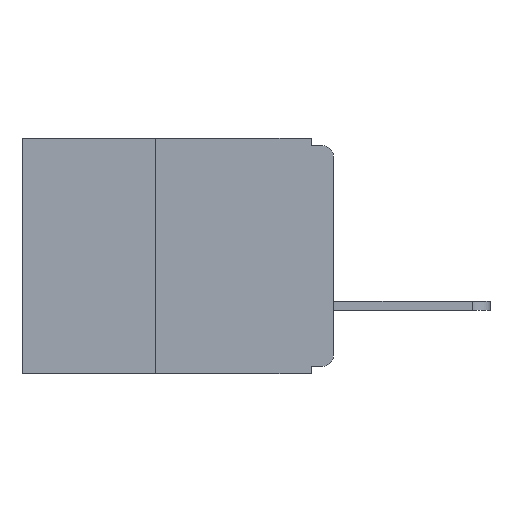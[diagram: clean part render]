
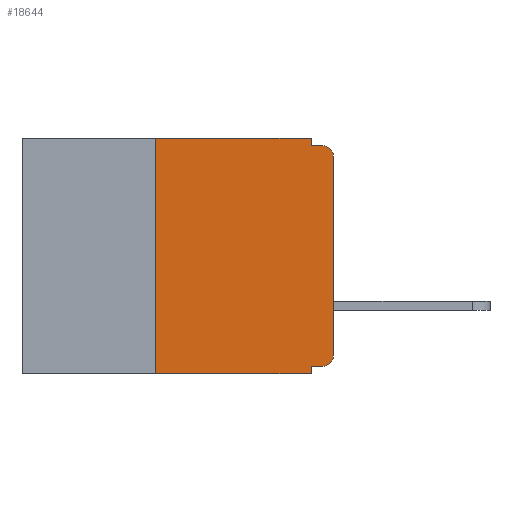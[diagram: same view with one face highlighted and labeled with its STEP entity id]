
A CAD part, left-side view. The second image highlights one B-rep face of the part: STEP entity #18644.
In plain terms, the highlighted planar face has unit normal (-1, 0, 0).
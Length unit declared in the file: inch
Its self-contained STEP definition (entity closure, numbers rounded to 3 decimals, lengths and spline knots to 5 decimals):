
#271 = VECTOR ( 'NONE', #26319, 39.37008 ) ;
#470 = EDGE_CURVE ( 'NONE', #30614, #11118, #21927, .T. ) ;
#960 = VECTOR ( 'NONE', #23253, 39.37008 ) ;
#1265 = VERTEX_POINT ( 'NONE', #15698 ) ;
#1333 = CARTESIAN_POINT ( 'NONE',  ( 0., 0.031, 0. ) ) ;
#3587 = DIRECTION ( 'NONE',  ( 0., 0., -1. ) ) ;
#4010 = DIRECTION ( 'NONE',  ( 0., 0., -1. ) ) ;
#4295 = EDGE_CURVE ( 'NONE', #5177, #17000, #7748, .T. ) ;
#4303 = CARTESIAN_POINT ( 'NONE',  ( 0., 0.015, -0.01 ) ) ;
#5177 = VERTEX_POINT ( 'NONE', #26913 ) ;
#5178 = LINE ( 'NONE', #8934, #17612 ) ;
#5213 = VECTOR ( 'NONE', #18638, 39.37008 ) ;
#6089 = CARTESIAN_POINT ( 'NONE',  ( 0., 0.031, -0.33 ) ) ;
#6335 = DIRECTION ( 'NONE',  ( 0., -1., 0. ) ) ;
#6690 = EDGE_CURVE ( 'NONE', #17000, #25596, #9589, .T. ) ;
#6810 = LINE ( 'NONE', #26213, #271 ) ;
#7748 = LINE ( 'NONE', #12153, #20123 ) ;
#7890 = EDGE_CURVE ( 'NONE', #17106, #25596, #20689, .T. ) ;
#8322 = FACE_OUTER_BOUND ( 'NONE', #29855, .T. ) ;
#8396 = CARTESIAN_POINT ( 'NONE',  ( 0., 0.25, -0.33 ) ) ;
#8934 = CARTESIAN_POINT ( 'NONE',  ( 0., 0.031, -0.33 ) ) ;
#9293 = ORIENTED_EDGE ( 'NONE', *, *, #21731, .T. ) ;
#9324 = CARTESIAN_POINT ( 'NONE',  ( 0., 0.015, -0.305 ) ) ;
#9589 = CIRCLE ( 'NONE', #30154, 0.015 ) ;
#10976 = CARTESIAN_POINT ( 'NONE',  ( 0., 0.437, 0. ) ) ;
#11118 = VERTEX_POINT ( 'NONE', #6089 ) ;
#11634 = LINE ( 'NONE', #28216, #24750 ) ;
#11778 = DIRECTION ( 'NONE',  ( 0., 0., -1. ) ) ;
#12010 = CARTESIAN_POINT ( 'NONE',  ( 0., 0.031, -0.32 ) ) ;
#12043 = DIRECTION ( 'NONE',  ( 0., 0., 1. ) ) ;
#12153 = CARTESIAN_POINT ( 'NONE',  ( 0., 0., 0. ) ) ;
#12366 = ORIENTED_EDGE ( 'NONE', *, *, #18767, .F. ) ;
#12863 = CARTESIAN_POINT ( 'NONE',  ( 0., 0.437, -0.33 ) ) ;
#13578 = DIRECTION ( 'NONE',  ( 0., -1., 0. ) ) ;
#13692 = CARTESIAN_POINT ( 'NONE',  ( 0., 0., -0.025 ) ) ;
#13906 = EDGE_CURVE ( 'NONE', #30614, #19021, #6810, .T. ) ;
#14145 = VECTOR ( 'NONE', #27816, 39.37008 ) ;
#14322 = AXIS2_PLACEMENT_3D ( 'NONE', #10976, #18439, #3587 ) ;
#14471 = EDGE_CURVE ( 'NONE', #1265, #17106, #24163, .T. ) ;
#14710 = CIRCLE ( 'NONE', #26013, 0.015 ) ;
#15698 = CARTESIAN_POINT ( 'NONE',  ( 0., 0.031, 0. ) ) ;
#17000 = VERTEX_POINT ( 'NONE', #13692 ) ;
#17106 = VERTEX_POINT ( 'NONE', #28732 ) ;
#17305 = DIRECTION ( 'NONE',  ( 0., 0., -1. ) ) ;
#17332 = DIRECTION ( 'NONE',  ( -1., 0., 0. ) ) ;
#17340 = CARTESIAN_POINT ( 'NONE',  ( 0., 0.015, -0.025 ) ) ;
#17612 = VECTOR ( 'NONE', #4010, 39.37008 ) ;
#18439 = DIRECTION ( 'NONE',  ( 1., 0., 0. ) ) ;
#18638 = DIRECTION ( 'NONE',  ( 0., 0., -1. ) ) ;
#18644 = ADVANCED_FACE ( 'NONE', ( #8322 ), #28015, .F. ) ;
#18678 = EDGE_CURVE ( 'NONE', #27408, #19941, #20684, .T. ) ;
#18767 = EDGE_CURVE ( 'NONE', #19941, #11118, #5178, .T. ) ;
#18834 = ORIENTED_EDGE ( 'NONE', *, *, #7890, .F. ) ;
#19021 = VERTEX_POINT ( 'NONE', #24743 ) ;
#19305 = ORIENTED_EDGE ( 'NONE', *, *, #13906, .F. ) ;
#19941 = VERTEX_POINT ( 'NONE', #12010 ) ;
#20123 = VECTOR ( 'NONE', #12043, 39.37008 ) ;
#20464 = ORIENTED_EDGE ( 'NONE', *, *, #18678, .F. ) ;
#20684 = LINE ( 'NONE', #28223, #960 ) ;
#20689 = LINE ( 'NONE', #28662, #14145 ) ;
#20929 = EDGE_CURVE ( 'NONE', #19021, #1265, #11634, .T. ) ;
#21731 = EDGE_CURVE ( 'NONE', #27408, #5177, #14710, .T. ) ;
#21927 = LINE ( 'NONE', #12863, #28352 ) ;
#23253 = DIRECTION ( 'NONE',  ( 0., 1., 0. ) ) ;
#24163 = LINE ( 'NONE', #1333, #5213 ) ;
#24640 = ORIENTED_EDGE ( 'NONE', *, *, #20929, .F. ) ;
#24743 = CARTESIAN_POINT ( 'NONE',  ( 0., 0.25, 0. ) ) ;
#24750 = VECTOR ( 'NONE', #13578, 39.37008 ) ;
#25596 = VERTEX_POINT ( 'NONE', #4303 ) ;
#26013 = AXIS2_PLACEMENT_3D ( 'NONE', #9324, #26512, #11778 ) ;
#26073 = ORIENTED_EDGE ( 'NONE', *, *, #4295, .T. ) ;
#26213 = CARTESIAN_POINT ( 'NONE',  ( 0., 0.25, -0.33 ) ) ;
#26319 = DIRECTION ( 'NONE',  ( 0., 0., 1. ) ) ;
#26512 = DIRECTION ( 'NONE',  ( -1., 0., 0. ) ) ;
#26913 = CARTESIAN_POINT ( 'NONE',  ( 0., 0., -0.305 ) ) ;
#27408 = VERTEX_POINT ( 'NONE', #29026 ) ;
#27816 = DIRECTION ( 'NONE',  ( 0., -1., 0. ) ) ;
#28015 = PLANE ( 'NONE',  #14322 ) ;
#28216 = CARTESIAN_POINT ( 'NONE',  ( 0., 0.437, 0. ) ) ;
#28223 = CARTESIAN_POINT ( 'NONE',  ( 0., 0., -0.32 ) ) ;
#28352 = VECTOR ( 'NONE', #6335, 39.37008 ) ;
#28662 = CARTESIAN_POINT ( 'NONE',  ( 0., 0., -0.01 ) ) ;
#28732 = CARTESIAN_POINT ( 'NONE',  ( 0., 0.031, -0.01 ) ) ;
#29026 = CARTESIAN_POINT ( 'NONE',  ( 0., 0.015, -0.32 ) ) ;
#29073 = ORIENTED_EDGE ( 'NONE', *, *, #6690, .T. ) ;
#29492 = ORIENTED_EDGE ( 'NONE', *, *, #14471, .F. ) ;
#29855 = EDGE_LOOP ( 'NONE', ( #26073, #29073, #18834, #29492, #24640, #19305, #31010, #12366, #20464, #9293 ) ) ;
#30154 = AXIS2_PLACEMENT_3D ( 'NONE', #17340, #17332, #17305 ) ;
#30614 = VERTEX_POINT ( 'NONE', #8396 ) ;
#31010 = ORIENTED_EDGE ( 'NONE', *, *, #470, .T. ) ;
